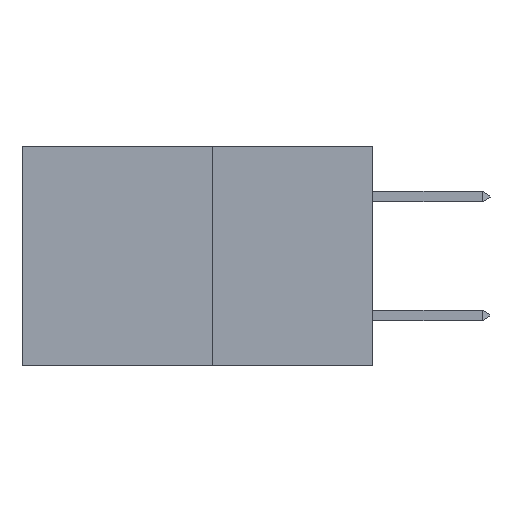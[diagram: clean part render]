
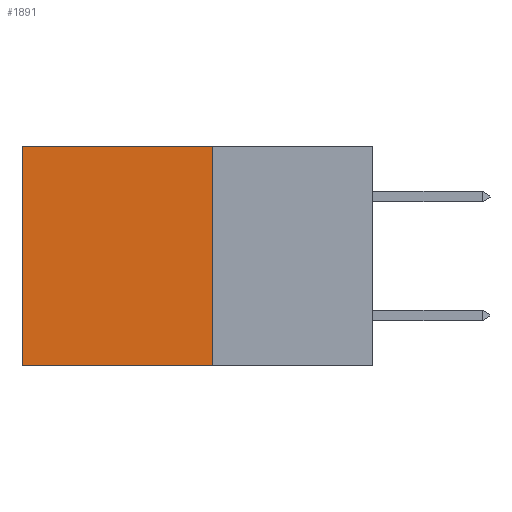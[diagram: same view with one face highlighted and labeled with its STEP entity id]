
A CAD part, left-side view. The second image highlights one B-rep face of the part: STEP entity #1891.
In plain terms, the highlighted planar face has unit normal (-1, 0, 0).
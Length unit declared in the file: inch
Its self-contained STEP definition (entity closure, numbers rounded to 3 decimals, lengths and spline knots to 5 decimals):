
#90 = DIRECTION ( 'NONE',  ( 1., 0., 0. ) ) ;
#700 = DIRECTION ( 'NONE',  ( 0., 1., 0. ) ) ;
#1193 = EDGE_CURVE ( 'NONE', #13063, #8507, #13445, .T. ) ;
#1213 = DIRECTION ( 'NONE',  ( 0., 0., -1. ) ) ;
#1374 = VECTOR ( 'NONE', #4244, 39.37008 ) ;
#1564 = FACE_OUTER_BOUND ( 'NONE', #14408, .T. ) ;
#1850 = PLANE ( 'NONE',  #4900 ) ;
#1891 = ADVANCED_FACE ( 'NONE', ( #1564 ), #1850, .F. ) ;
#1946 = CARTESIAN_POINT ( 'NONE',  ( 0.277, 0.27, 0. ) ) ;
#2404 = ORIENTED_EDGE ( 'NONE', *, *, #1193, .F. ) ;
#3737 = ORIENTED_EDGE ( 'NONE', *, *, #4545, .T. ) ;
#3789 = DIRECTION ( 'NONE',  ( 0., 0., -1. ) ) ;
#3928 = CARTESIAN_POINT ( 'NONE',  ( 0.277, 0.27, 0. ) ) ;
#4244 = DIRECTION ( 'NONE',  ( 0., 0., -1. ) ) ;
#4269 = CARTESIAN_POINT ( 'NONE',  ( 0.277, 0.59, 0. ) ) ;
#4381 = VECTOR ( 'NONE', #700, 39.37008 ) ;
#4545 = EDGE_CURVE ( 'NONE', #7586, #10976, #5487, .T. ) ;
#4900 = AXIS2_PLACEMENT_3D ( 'NONE', #9790, #90, #1213 ) ;
#5487 = LINE ( 'NONE', #8955, #6742 ) ;
#5525 = CARTESIAN_POINT ( 'NONE',  ( 0.277, 0.27, -0.37 ) ) ;
#6742 = VECTOR ( 'NONE', #3789, 39.37008 ) ;
#7313 = DIRECTION ( 'NONE',  ( 0., 1., 0. ) ) ;
#7338 = CARTESIAN_POINT ( 'NONE',  ( 0.277, 0.27, -0.37 ) ) ;
#7586 = VERTEX_POINT ( 'NONE', #4269 ) ;
#8159 = ORIENTED_EDGE ( 'NONE', *, *, #10770, .T. ) ;
#8507 = VERTEX_POINT ( 'NONE', #10271 ) ;
#8875 = CARTESIAN_POINT ( 'NONE',  ( 0.277, 0.59, -0.37 ) ) ;
#8955 = CARTESIAN_POINT ( 'NONE',  ( 0.277, 0.59, -0.37 ) ) ;
#9790 = CARTESIAN_POINT ( 'NONE',  ( 0.277, 0.27, -0.37 ) ) ;
#10271 = CARTESIAN_POINT ( 'NONE',  ( 0.277, 0.27, -0.37 ) ) ;
#10770 = EDGE_CURVE ( 'NONE', #13063, #7586, #15054, .T. ) ;
#10976 = VERTEX_POINT ( 'NONE', #8875 ) ;
#11385 = LINE ( 'NONE', #7338, #4381 ) ;
#11724 = VECTOR ( 'NONE', #7313, 39.37008 ) ;
#12750 = ORIENTED_EDGE ( 'NONE', *, *, #14846, .F. ) ;
#13063 = VERTEX_POINT ( 'NONE', #3928 ) ;
#13445 = LINE ( 'NONE', #5525, #1374 ) ;
#14408 = EDGE_LOOP ( 'NONE', ( #3737, #12750, #2404, #8159 ) ) ;
#14846 = EDGE_CURVE ( 'NONE', #8507, #10976, #11385, .T. ) ;
#15054 = LINE ( 'NONE', #1946, #11724 ) ;
